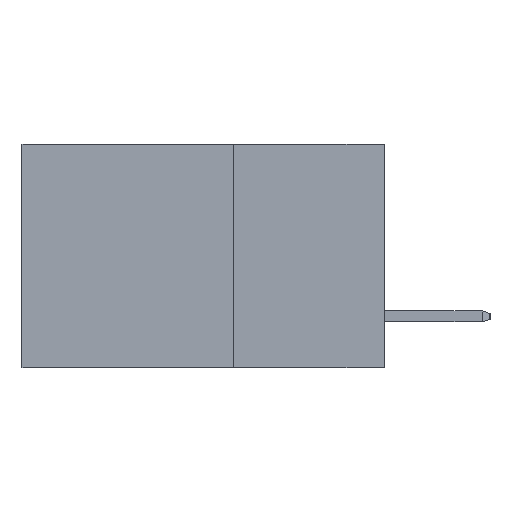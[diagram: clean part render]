
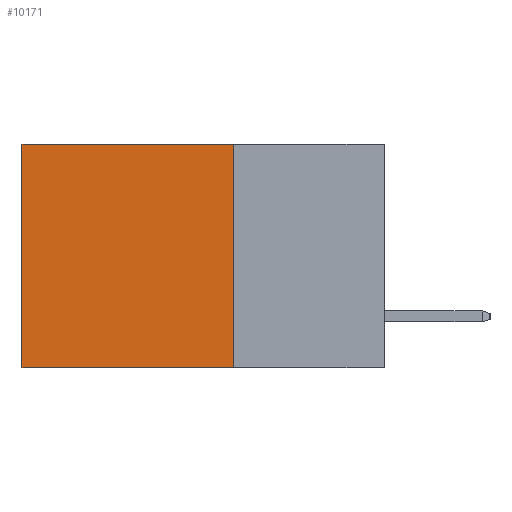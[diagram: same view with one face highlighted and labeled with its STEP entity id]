
A CAD part, left-side view. The second image highlights one B-rep face of the part: STEP entity #10171.
In plain terms, the highlighted planar face has unit normal (-1, 0, 0).
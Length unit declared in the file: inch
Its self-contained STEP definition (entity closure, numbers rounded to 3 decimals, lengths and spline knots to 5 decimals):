
#381 = VECTOR ( 'NONE', #13764, 39.37008 ) ;
#1241 = PLANE ( 'NONE',  #9036 ) ;
#1741 = CARTESIAN_POINT ( 'NONE',  ( 0.298, 0.25, 0. ) ) ;
#1849 = EDGE_CURVE ( 'NONE', #3783, #16749, #3943, .T. ) ;
#3783 = VERTEX_POINT ( 'NONE', #9525 ) ;
#3943 = LINE ( 'NONE', #9100, #381 ) ;
#4105 = ORIENTED_EDGE ( 'NONE', *, *, #5033, .F. ) ;
#4167 = CARTESIAN_POINT ( 'NONE',  ( 0.298, 0.6, 0. ) ) ;
#4286 = DIRECTION ( 'NONE',  ( 1., 0., 0. ) ) ;
#4795 = VERTEX_POINT ( 'NONE', #13466 ) ;
#5033 = EDGE_CURVE ( 'NONE', #4795, #6473, #15596, .T. ) ;
#5708 = FACE_OUTER_BOUND ( 'NONE', #16241, .T. ) ;
#6193 = DIRECTION ( 'NONE',  ( 0., 0., -1. ) ) ;
#6473 = VERTEX_POINT ( 'NONE', #14870 ) ;
#7220 = CARTESIAN_POINT ( 'NONE',  ( 0.298, 0.25, 0. ) ) ;
#7939 = ORIENTED_EDGE ( 'NONE', *, *, #1849, .T. ) ;
#9036 = AXIS2_PLACEMENT_3D ( 'NONE', #7220, #4286, #14542 ) ;
#9100 = CARTESIAN_POINT ( 'NONE',  ( 0.298, 0.25, 0. ) ) ;
#9322 = EDGE_CURVE ( 'NONE', #3783, #4795, #17657, .T. ) ;
#9525 = CARTESIAN_POINT ( 'NONE',  ( 0.298, 0.25, 0. ) ) ;
#9623 = CARTESIAN_POINT ( 'NONE',  ( 0.298, 0.25, -0.37 ) ) ;
#9848 = VECTOR ( 'NONE', #6193, 39.37008 ) ;
#10171 = ADVANCED_FACE ( 'NONE', ( #5708 ), #1241, .F. ) ;
#10359 = EDGE_CURVE ( 'NONE', #16749, #6473, #13734, .T. ) ;
#10831 = ORIENTED_EDGE ( 'NONE', *, *, #10359, .T. ) ;
#12575 = DIRECTION ( 'NONE',  ( 0., 1., 0. ) ) ;
#13466 = CARTESIAN_POINT ( 'NONE',  ( 0.298, 0.25, -0.37 ) ) ;
#13734 = LINE ( 'NONE', #16312, #9848 ) ;
#13764 = DIRECTION ( 'NONE',  ( 0., 1., 0. ) ) ;
#14342 = VECTOR ( 'NONE', #17841, 39.37008 ) ;
#14542 = DIRECTION ( 'NONE',  ( 0., 0., -1. ) ) ;
#14870 = CARTESIAN_POINT ( 'NONE',  ( 0.298, 0.6, -0.37 ) ) ;
#15596 = LINE ( 'NONE', #9623, #18942 ) ;
#16241 = EDGE_LOOP ( 'NONE', ( #10831, #4105, #17865, #7939 ) ) ;
#16312 = CARTESIAN_POINT ( 'NONE',  ( 0.298, 0.6, 0. ) ) ;
#16749 = VERTEX_POINT ( 'NONE', #4167 ) ;
#17657 = LINE ( 'NONE', #1741, #14342 ) ;
#17841 = DIRECTION ( 'NONE',  ( 0., 0., -1. ) ) ;
#17865 = ORIENTED_EDGE ( 'NONE', *, *, #9322, .F. ) ;
#18942 = VECTOR ( 'NONE', #12575, 39.37008 ) ;
